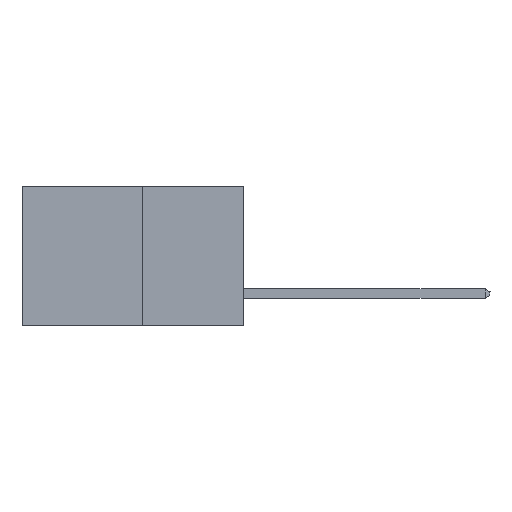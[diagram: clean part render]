
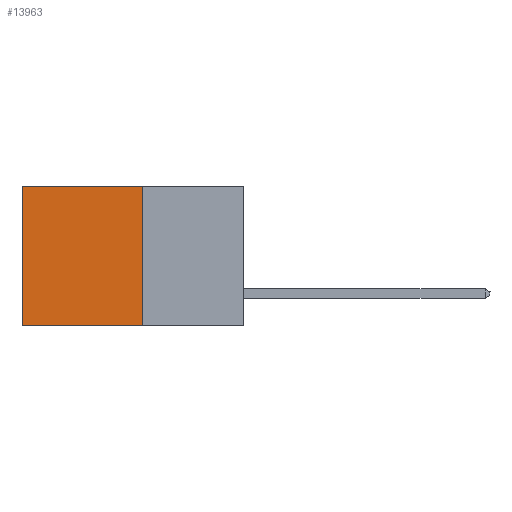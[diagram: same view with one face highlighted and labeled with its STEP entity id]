
A CAD part, left-side view. The second image highlights one B-rep face of the part: STEP entity #13963.
In plain terms, the highlighted planar face has unit normal (-1, 0, 0).
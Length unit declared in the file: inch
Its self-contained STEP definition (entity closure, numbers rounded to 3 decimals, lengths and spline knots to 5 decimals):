
#520 = LINE ( 'NONE', #1628, #11792 ) ;
#621 = CARTESIAN_POINT ( 'NONE',  ( 0.277, 0.27, 0. ) ) ;
#653 = EDGE_CURVE ( 'NONE', #11636, #15302, #7434, .T. ) ;
#1123 = AXIS2_PLACEMENT_3D ( 'NONE', #10306, #10364, #1578 ) ;
#1553 = FACE_OUTER_BOUND ( 'NONE', #2925, .T. ) ;
#1578 = DIRECTION ( 'NONE',  ( 0., 0., -1. ) ) ;
#1628 = CARTESIAN_POINT ( 'NONE',  ( 0.277, 0.27, -0.37 ) ) ;
#2105 = ORIENTED_EDGE ( 'NONE', *, *, #18060, .F. ) ;
#2323 = DIRECTION ( 'NONE',  ( 0., 1., 0. ) ) ;
#2626 = CARTESIAN_POINT ( 'NONE',  ( 0.277, 0.27, 0. ) ) ;
#2925 = EDGE_LOOP ( 'NONE', ( #3898, #16242, #2105, #17580 ) ) ;
#3092 = DIRECTION ( 'NONE',  ( 0., 1., 0. ) ) ;
#3898 = ORIENTED_EDGE ( 'NONE', *, *, #6685, .T. ) ;
#4947 = CARTESIAN_POINT ( 'NONE',  ( 0.277, 0.59, -0.37 ) ) ;
#4953 = CARTESIAN_POINT ( 'NONE',  ( 0.277, 0.27, -0.37 ) ) ;
#6685 = EDGE_CURVE ( 'NONE', #15302, #12169, #17998, .T. ) ;
#7278 = VECTOR ( 'NONE', #10736, 39.37008 ) ;
#7434 = LINE ( 'NONE', #2626, #11354 ) ;
#8539 = VERTEX_POINT ( 'NONE', #4953 ) ;
#8865 = PLANE ( 'NONE',  #1123 ) ;
#8946 = CARTESIAN_POINT ( 'NONE',  ( 0.277, 0.59, 0. ) ) ;
#8974 = DIRECTION ( 'NONE',  ( 0., 0., -1. ) ) ;
#10306 = CARTESIAN_POINT ( 'NONE',  ( 0.277, 0.27, -0.37 ) ) ;
#10364 = DIRECTION ( 'NONE',  ( 1., 0., 0. ) ) ;
#10484 = LINE ( 'NONE', #13346, #14319 ) ;
#10736 = DIRECTION ( 'NONE',  ( 0., 0., -1. ) ) ;
#11354 = VECTOR ( 'NONE', #2323, 39.37008 ) ;
#11636 = VERTEX_POINT ( 'NONE', #621 ) ;
#11792 = VECTOR ( 'NONE', #8974, 39.37008 ) ;
#12169 = VERTEX_POINT ( 'NONE', #12278 ) ;
#12278 = CARTESIAN_POINT ( 'NONE',  ( 0.277, 0.59, -0.37 ) ) ;
#13346 = CARTESIAN_POINT ( 'NONE',  ( 0.277, 0.27, -0.37 ) ) ;
#13963 = ADVANCED_FACE ( 'NONE', ( #1553 ), #8865, .F. ) ;
#14319 = VECTOR ( 'NONE', #3092, 39.37008 ) ;
#15302 = VERTEX_POINT ( 'NONE', #8946 ) ;
#16242 = ORIENTED_EDGE ( 'NONE', *, *, #16845, .F. ) ;
#16845 = EDGE_CURVE ( 'NONE', #8539, #12169, #10484, .T. ) ;
#17580 = ORIENTED_EDGE ( 'NONE', *, *, #653, .T. ) ;
#17998 = LINE ( 'NONE', #4947, #7278 ) ;
#18060 = EDGE_CURVE ( 'NONE', #11636, #8539, #520, .T. ) ;
